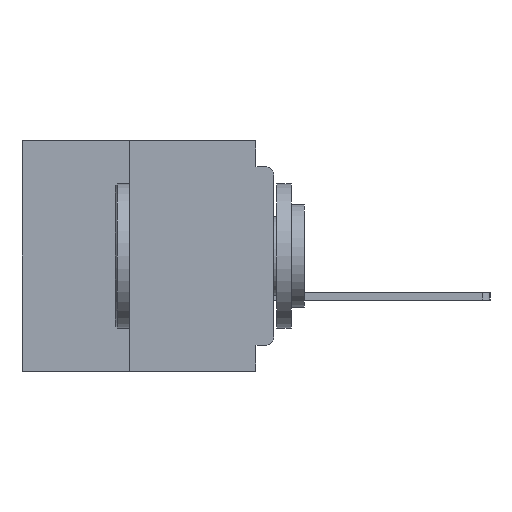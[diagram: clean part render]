
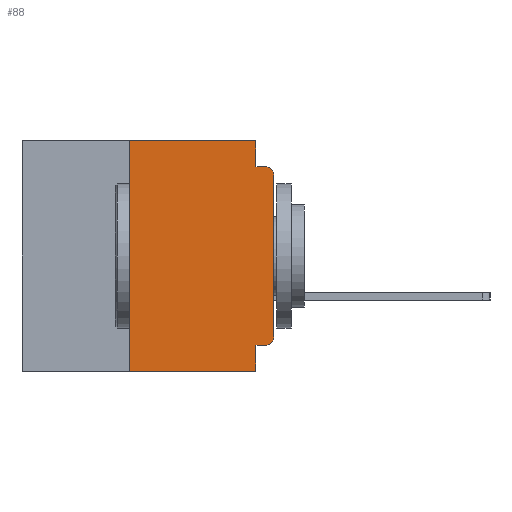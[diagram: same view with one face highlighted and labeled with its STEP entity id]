
A CAD part, left-side view. The second image highlights one B-rep face of the part: STEP entity #88.
In plain terms, the highlighted planar face has unit normal (-1, 0, 0).
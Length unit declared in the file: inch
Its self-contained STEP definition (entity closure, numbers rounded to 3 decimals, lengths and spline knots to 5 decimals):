
#88 = ADVANCED_FACE ( 'NONE', ( #29019 ), #60178, .F. ) ;
#410 = DIRECTION ( 'NONE',  ( 0., 1., 0. ) ) ;
#1344 = ORIENTED_EDGE ( 'NONE', *, *, #58037, .T. ) ;
#1638 = CARTESIAN_POINT ( 'NONE',  ( 0., 0.25, -0.4 ) ) ;
#2582 = LINE ( 'NONE', #36269, #26941 ) ;
#3225 = CARTESIAN_POINT ( 'NONE',  ( 0., 0.437, 0. ) ) ;
#3800 = ORIENTED_EDGE ( 'NONE', *, *, #52776, .F. ) ;
#4835 = VERTEX_POINT ( 'NONE', #35812 ) ;
#5117 = VECTOR ( 'NONE', #410, 39.37008 ) ;
#5984 = VERTEX_POINT ( 'NONE', #54766 ) ;
#6691 = VECTOR ( 'NONE', #36522, 39.37008 ) ;
#6781 = CARTESIAN_POINT ( 'NONE',  ( 0., 0.031, -0.4 ) ) ;
#7000 = VERTEX_POINT ( 'NONE', #62749 ) ;
#8264 = CARTESIAN_POINT ( 'NONE',  ( 0., 0., -0.045 ) ) ;
#8471 = EDGE_LOOP ( 'NONE', ( #1344, #8623, #28060, #9299, #27122, #56178, #23260, #59266, #3800, #21117 ) ) ;
#8623 = ORIENTED_EDGE ( 'NONE', *, *, #47073, .T. ) ;
#8729 = VERTEX_POINT ( 'NONE', #22707 ) ;
#9299 = ORIENTED_EDGE ( 'NONE', *, *, #41547, .F. ) ;
#13567 = VERTEX_POINT ( 'NONE', #45837 ) ;
#14003 = DIRECTION ( 'NONE',  ( -1., 0., 0. ) ) ;
#15648 = DIRECTION ( 'NONE',  ( -1., 0., 0. ) ) ;
#15927 = EDGE_CURVE ( 'NONE', #58690, #55044, #41539, .T. ) ;
#16347 = LINE ( 'NONE', #8264, #53635 ) ;
#16664 = VECTOR ( 'NONE', #34270, 39.37008 ) ;
#17922 = DIRECTION ( 'NONE',  ( 0., -1., 0. ) ) ;
#18481 = EDGE_CURVE ( 'NONE', #7000, #5984, #58533, .T. ) ;
#20453 = VECTOR ( 'NONE', #21260, 39.37008 ) ;
#21117 = ORIENTED_EDGE ( 'NONE', *, *, #18481, .T. ) ;
#21260 = DIRECTION ( 'NONE',  ( 0., 0., -1. ) ) ;
#22180 = AXIS2_PLACEMENT_3D ( 'NONE', #44785, #15648, #49687 ) ;
#22261 = CARTESIAN_POINT ( 'NONE',  ( 0., 0.437, -0.4 ) ) ;
#22707 = CARTESIAN_POINT ( 'NONE',  ( 0., 0., -0.06 ) ) ;
#23260 = ORIENTED_EDGE ( 'NONE', *, *, #25484, .T. ) ;
#25484 = EDGE_CURVE ( 'NONE', #61458, #33891, #43487, .T. ) ;
#26504 = DIRECTION ( 'NONE',  ( 0., 0., 1. ) ) ;
#26941 = VECTOR ( 'NONE', #26504, 39.37008 ) ;
#27122 = ORIENTED_EDGE ( 'NONE', *, *, #15927, .F. ) ;
#27610 = DIRECTION ( 'NONE',  ( 0., -1., 0. ) ) ;
#28060 = ORIENTED_EDGE ( 'NONE', *, *, #54828, .F. ) ;
#28615 = VECTOR ( 'NONE', #17922, 39.37008 ) ;
#29019 = FACE_OUTER_BOUND ( 'NONE', #8471, .T. ) ;
#29365 = CARTESIAN_POINT ( 'NONE',  ( 0., 0., 0. ) ) ;
#29451 = LINE ( 'NONE', #34466, #5117 ) ;
#29603 = LINE ( 'NONE', #29365, #16664 ) ;
#30732 = AXIS2_PLACEMENT_3D ( 'NONE', #43109, #14003, #48032 ) ;
#31301 = EDGE_CURVE ( 'NONE', #13567, #33891, #47848, .T. ) ;
#31311 = CIRCLE ( 'NONE', #22180, 0.015 ) ;
#31546 = CARTESIAN_POINT ( 'NONE',  ( 0., 0.031, -0.4 ) ) ;
#32378 = VERTEX_POINT ( 'NONE', #53643 ) ;
#33891 = VERTEX_POINT ( 'NONE', #31546 ) ;
#34270 = DIRECTION ( 'NONE',  ( 0., 0., 1. ) ) ;
#34466 = CARTESIAN_POINT ( 'NONE',  ( 0., 0., -0.355 ) ) ;
#35812 = CARTESIAN_POINT ( 'NONE',  ( 0., 0.015, -0.045 ) ) ;
#36269 = CARTESIAN_POINT ( 'NONE',  ( 0., 0.25, -0.4 ) ) ;
#36522 = DIRECTION ( 'NONE',  ( 0., 0., -1. ) ) ;
#38854 = CARTESIAN_POINT ( 'NONE',  ( 0., 0.031, 0. ) ) ;
#41539 = LINE ( 'NONE', #3225, #28615 ) ;
#41547 = EDGE_CURVE ( 'NONE', #55044, #32378, #62997, .T. ) ;
#43109 = CARTESIAN_POINT ( 'NONE',  ( 0., 0.015, -0.34 ) ) ;
#43487 = LINE ( 'NONE', #22261, #45009 ) ;
#44785 = CARTESIAN_POINT ( 'NONE',  ( 0., 0.015, -0.06 ) ) ;
#45009 = VECTOR ( 'NONE', #56236, 39.37008 ) ;
#45837 = CARTESIAN_POINT ( 'NONE',  ( 0., 0.031, -0.355 ) ) ;
#47073 = EDGE_CURVE ( 'NONE', #8729, #4835, #31311, .T. ) ;
#47848 = LINE ( 'NONE', #6781, #20453 ) ;
#48032 = DIRECTION ( 'NONE',  ( 0., 0., -1. ) ) ;
#48446 = AXIS2_PLACEMENT_3D ( 'NONE', #59501, #59004, #58924 ) ;
#48955 = EDGE_CURVE ( 'NONE', #61458, #58690, #2582, .T. ) ;
#49687 = DIRECTION ( 'NONE',  ( 0., 0., -1. ) ) ;
#52349 = CARTESIAN_POINT ( 'NONE',  ( 0., 0.25, 0. ) ) ;
#52776 = EDGE_CURVE ( 'NONE', #7000, #13567, #29451, .T. ) ;
#53635 = VECTOR ( 'NONE', #27610, 39.37008 ) ;
#53643 = CARTESIAN_POINT ( 'NONE',  ( 0., 0.031, -0.045 ) ) ;
#54766 = CARTESIAN_POINT ( 'NONE',  ( 0., 0., -0.34 ) ) ;
#54828 = EDGE_CURVE ( 'NONE', #32378, #4835, #16347, .T. ) ;
#55044 = VERTEX_POINT ( 'NONE', #38854 ) ;
#56178 = ORIENTED_EDGE ( 'NONE', *, *, #48955, .F. ) ;
#56236 = DIRECTION ( 'NONE',  ( 0., -1., 0. ) ) ;
#58037 = EDGE_CURVE ( 'NONE', #5984, #8729, #29603, .T. ) ;
#58533 = CIRCLE ( 'NONE', #30732, 0.015 ) ;
#58690 = VERTEX_POINT ( 'NONE', #52349 ) ;
#58924 = DIRECTION ( 'NONE',  ( 0., 0., -1. ) ) ;
#59004 = DIRECTION ( 'NONE',  ( 1., 0., 0. ) ) ;
#59266 = ORIENTED_EDGE ( 'NONE', *, *, #31301, .F. ) ;
#59501 = CARTESIAN_POINT ( 'NONE',  ( 0., 0.437, 0. ) ) ;
#60178 = PLANE ( 'NONE',  #48446 ) ;
#60742 = CARTESIAN_POINT ( 'NONE',  ( 0., 0.031, 0. ) ) ;
#61458 = VERTEX_POINT ( 'NONE', #1638 ) ;
#62749 = CARTESIAN_POINT ( 'NONE',  ( 0., 0.015, -0.355 ) ) ;
#62997 = LINE ( 'NONE', #60742, #6691 ) ;
